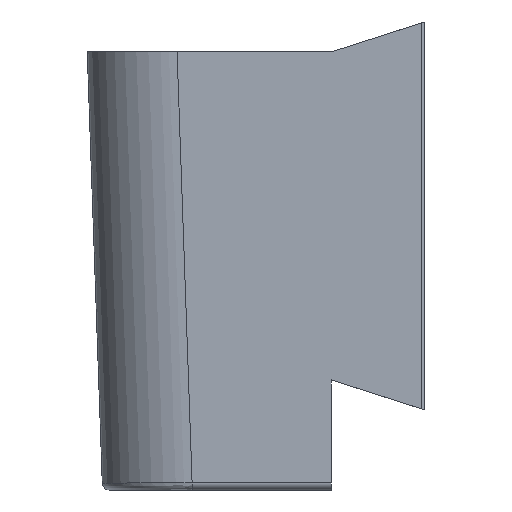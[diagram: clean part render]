
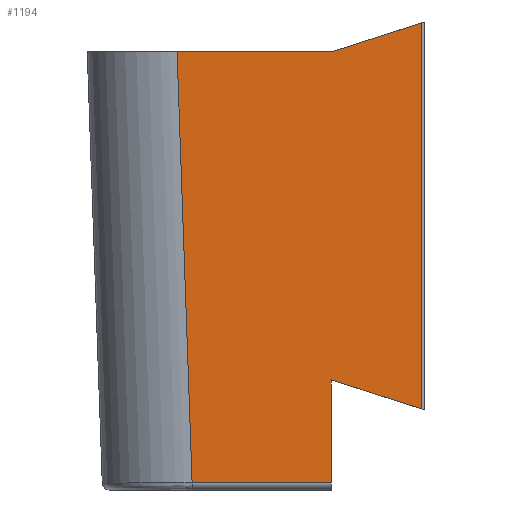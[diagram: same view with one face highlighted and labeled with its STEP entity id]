
A CAD part, left-side view. The second image highlights one B-rep face of the part: STEP entity #1194.
In plain terms, the highlighted planar face has unit normal (-1, 0, 0).
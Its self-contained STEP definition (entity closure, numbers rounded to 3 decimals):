
#7 = AXIS2_PLACEMENT_3D ( 'NONE', #892, #217, #792 ) ;
#35 = VECTOR ( 'NONE', #1095, 1000. ) ;
#125 = VERTEX_POINT ( 'NONE', #1126 ) ;
#129 = CARTESIAN_POINT ( 'NONE',  ( -8.001, -1.6, 0.528 ) ) ;
#149 = DIRECTION ( 'NONE',  ( 0., -0.035, -0.999 ) ) ;
#162 = VERTEX_POINT ( 'NONE', #221 ) ;
#163 = CARTESIAN_POINT ( 'NONE',  ( -8.001, 2.463, -7.62 ) ) ;
#194 = LINE ( 'NONE', #1148, #35 ) ;
#200 = DIRECTION ( 'NONE',  ( 0., 0., -1. ) ) ;
#217 = DIRECTION ( 'NONE',  ( -1., 0., 0. ) ) ;
#221 = CARTESIAN_POINT ( 'NONE',  ( -8.001, 0., -7.62 ) ) ;
#238 = VERTEX_POINT ( 'NONE', #1042 ) ;
#298 = EDGE_CURVE ( 'NONE', #238, #1125, #194, .T. ) ;
#333 = EDGE_CURVE ( 'NONE', #1252, #162, #1093, .T. ) ;
#383 = CARTESIAN_POINT ( 'NONE',  ( -8.001, 0., -7.747 ) ) ;
#402 = PLANE ( 'NONE',  #7 ) ;
#431 = ORIENTED_EDGE ( 'NONE', *, *, #333, .T. ) ;
#455 = VERTEX_POINT ( 'NONE', #669 ) ;
#462 = EDGE_CURVE ( 'NONE', #455, #162, #684, .T. ) ;
#547 = CARTESIAN_POINT ( 'NONE',  ( -8.001, -1.6, 0.512 ) ) ;
#562 = DIRECTION ( 'NONE',  ( 0., 0.952, 0.305 ) ) ;
#574 = ORIENTED_EDGE ( 'NONE', *, *, #298, .F. ) ;
#575 = EDGE_CURVE ( 'NONE', #125, #1125, #952, .T. ) ;
#594 = EDGE_CURVE ( 'NONE', #1047, #1252, #980, .T. ) ;
#621 = ORIENTED_EDGE ( 'NONE', *, *, #999, .F. ) ;
#655 = DIRECTION ( 'NONE',  ( 0., -1., 0. ) ) ;
#669 = CARTESIAN_POINT ( 'NONE',  ( -8.001, 0., -5.801 ) ) ;
#670 = EDGE_LOOP ( 'NONE', ( #776, #431, #747, #621, #752, #574, #866 ) ) ;
#684 = LINE ( 'NONE', #383, #1010 ) ;
#709 = FACE_OUTER_BOUND ( 'NONE', #670, .T. ) ;
#722 = CARTESIAN_POINT ( 'NONE',  ( -8.001, 2.461, -7.692 ) ) ;
#747 = ORIENTED_EDGE ( 'NONE', *, *, #462, .F. ) ;
#752 = ORIENTED_EDGE ( 'NONE', *, *, #575, .T. ) ;
#776 = ORIENTED_EDGE ( 'NONE', *, *, #594, .T. ) ;
#790 = VECTOR ( 'NONE', #655, 1000. ) ;
#792 = DIRECTION ( 'NONE',  ( 0., 0., 1. ) ) ;
#796 = CARTESIAN_POINT ( 'NONE',  ( -8.001, 4.318, 0. ) ) ;
#849 = DIRECTION ( 'NONE',  ( 0., -1., 0. ) ) ;
#859 = CARTESIAN_POINT ( 'NONE',  ( -8.001, 0., -7.62 ) ) ;
#865 = VECTOR ( 'NONE', #149, 1000. ) ;
#866 = ORIENTED_EDGE ( 'NONE', *, *, #1055, .F. ) ;
#892 = CARTESIAN_POINT ( 'NONE',  ( -8.001, -1.651, 0. ) ) ;
#912 = VECTOR ( 'NONE', #562, 1000. ) ;
#913 = VECTOR ( 'NONE', #849, 1000. ) ;
#933 = VECTOR ( 'NONE', #1147, 1000. ) ;
#951 = CARTESIAN_POINT ( 'NONE',  ( -8.001, 2.73, 0. ) ) ;
#952 = LINE ( 'NONE', #129, #933 ) ;
#980 = LINE ( 'NONE', #722, #865 ) ;
#999 = EDGE_CURVE ( 'NONE', #125, #455, #1221, .T. ) ;
#1010 = VECTOR ( 'NONE', #200, 1000. ) ;
#1042 = CARTESIAN_POINT ( 'NONE',  ( -8.001, 0., 0. ) ) ;
#1047 = VERTEX_POINT ( 'NONE', #951 ) ;
#1055 = EDGE_CURVE ( 'NONE', #1047, #238, #1177, .T. ) ;
#1093 = LINE ( 'NONE', #859, #790 ) ;
#1095 = DIRECTION ( 'NONE',  ( 0., -0.952, 0.305 ) ) ;
#1125 = VERTEX_POINT ( 'NONE', #547 ) ;
#1126 = CARTESIAN_POINT ( 'NONE',  ( -8.001, -1.6, -6.313 ) ) ;
#1147 = DIRECTION ( 'NONE',  ( 0., 0., 1. ) ) ;
#1148 = CARTESIAN_POINT ( 'NONE',  ( -8.001, -1.651, 0.528 ) ) ;
#1177 = LINE ( 'NONE', #796, #913 ) ;
#1194 = ADVANCED_FACE ( 'NONE', ( #709 ), #402, .T. ) ;
#1221 = LINE ( 'NONE', #1284, #912 ) ;
#1252 = VERTEX_POINT ( 'NONE', #163 ) ;
#1284 = CARTESIAN_POINT ( 'NONE',  ( -8.001, 0., -5.801 ) ) ;
